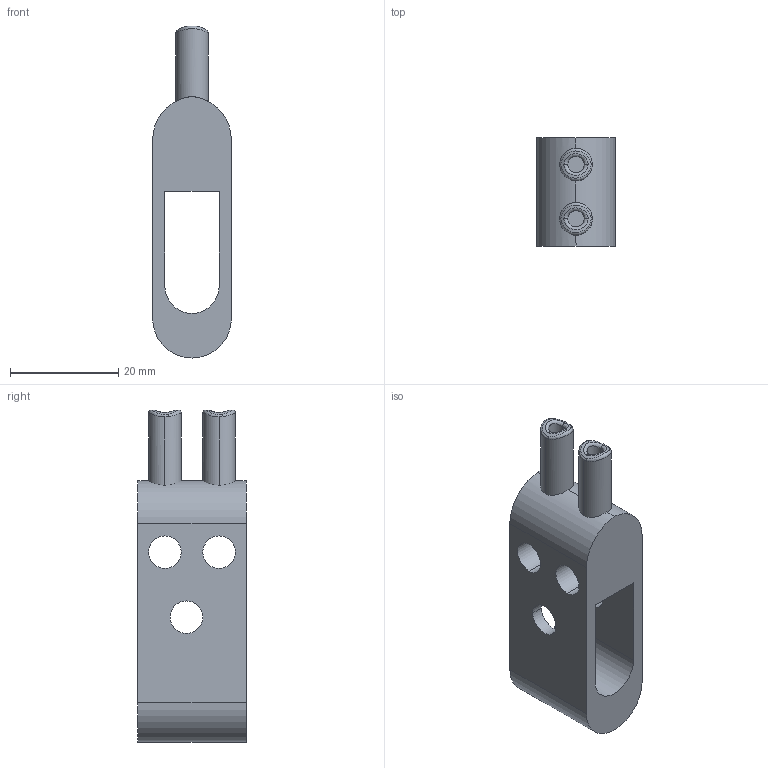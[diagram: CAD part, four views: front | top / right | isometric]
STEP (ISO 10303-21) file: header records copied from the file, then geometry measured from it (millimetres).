
FILE_DESCRIPTION (( 'STEP AP214' ), '1' );
FILE_NAME ('Trigger_Carriage.step', '2014-05-14T06:09:20', ( 'WarFairy' ), ( '' ), 'SwSTEP 2.0', 'SolidWorks 2013', '' );
FILE_SCHEMA (( 'AUTOMOTIVE_DESIGN' ));
Length unit declared in the file: inch
Products named in the file (1): Trigger_Carriage
Bounding box: 14.5 x 20 x 61.21 mm (x, y, z)
Volume: 8452.9 mm3; surface area: 5271.4 mm2
Topology: 1 solids, 1 shells, 40 faces, 108 edges, 72 vertices
Faces by surface type: cylinder 23, plane 9, bspline 8
Entity records: 4016 total; most frequent: CARTESIAN_POINT 3035, ORIENTED_EDGE 216, DIRECTION 164, EDGE_CURVE 108, VERTEX_POINT 72, AXIS2_PLACEMENT_3D 63, EDGE_LOOP 52, ADVANCED_FACE 40
